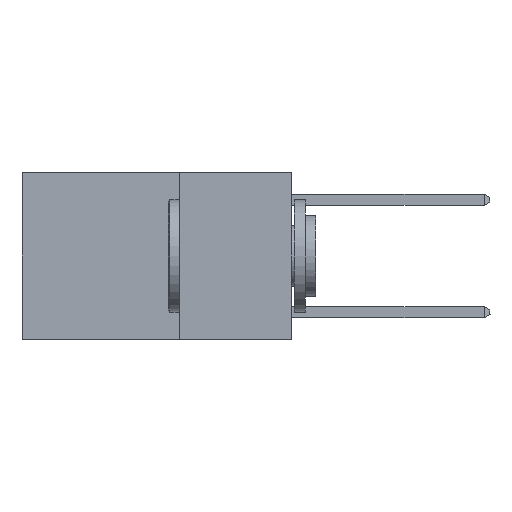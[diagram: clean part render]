
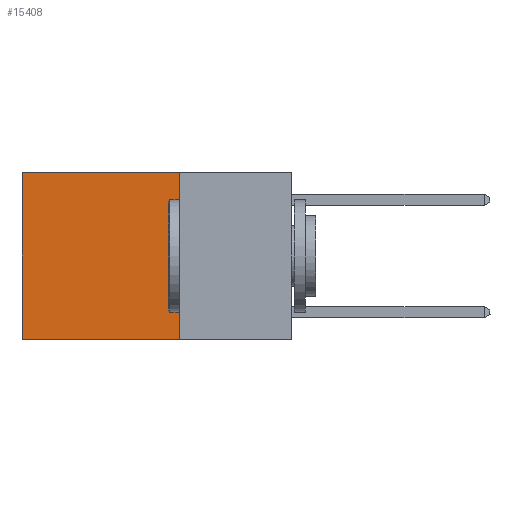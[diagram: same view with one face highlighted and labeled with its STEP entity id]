
A CAD part, left-side view. The second image highlights one B-rep face of the part: STEP entity #15408.
In plain terms, the highlighted planar face has unit normal (-1, 0, 0).
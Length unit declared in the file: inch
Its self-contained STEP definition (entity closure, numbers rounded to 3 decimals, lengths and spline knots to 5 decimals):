
#282 = VERTEX_POINT ( 'NONE', #19405 ) ;
#1904 = CARTESIAN_POINT ( 'NONE',  ( 0.2625, 0.25, -0.37 ) ) ;
#2249 = VECTOR ( 'NONE', #3381, 39.37008 ) ;
#2272 = LINE ( 'NONE', #5291, #2249 ) ;
#2725 = VERTEX_POINT ( 'NONE', #8084 ) ;
#3132 = VECTOR ( 'NONE', #20095, 39.37008 ) ;
#3381 = DIRECTION ( 'NONE',  ( 0., 0., -1. ) ) ;
#3656 = ORIENTED_EDGE ( 'NONE', *, *, #12179, .T. ) ;
#4263 = DIRECTION ( 'NONE',  ( 0., 0., -1. ) ) ;
#4786 = FACE_OUTER_BOUND ( 'NONE', #16411, .T. ) ;
#5291 = CARTESIAN_POINT ( 'NONE',  ( 0.2625, 0.6, 0. ) ) ;
#6138 = EDGE_CURVE ( 'NONE', #8339, #2725, #2272, .T. ) ;
#7059 = CARTESIAN_POINT ( 'NONE',  ( 0.2625, 0.25, 0. ) ) ;
#7097 = EDGE_CURVE ( 'NONE', #7276, #282, #9779, .T. ) ;
#7276 = VERTEX_POINT ( 'NONE', #9679 ) ;
#8084 = CARTESIAN_POINT ( 'NONE',  ( 0.2625, 0.6, -0.37 ) ) ;
#8153 = LINE ( 'NONE', #1904, #3132 ) ;
#8339 = VERTEX_POINT ( 'NONE', #14034 ) ;
#9037 = ORIENTED_EDGE ( 'NONE', *, *, #17999, .F. ) ;
#9679 = CARTESIAN_POINT ( 'NONE',  ( 0.2625, 0.25, 0. ) ) ;
#9779 = LINE ( 'NONE', #14354, #9848 ) ;
#9848 = VECTOR ( 'NONE', #4263, 39.37008 ) ;
#10473 = DIRECTION ( 'NONE',  ( 0., 0., -1. ) ) ;
#11497 = ORIENTED_EDGE ( 'NONE', *, *, #7097, .F. ) ;
#12179 = EDGE_CURVE ( 'NONE', #7276, #8339, #17061, .T. ) ;
#13060 = ORIENTED_EDGE ( 'NONE', *, *, #6138, .T. ) ;
#14034 = CARTESIAN_POINT ( 'NONE',  ( 0.2625, 0.6, 0. ) ) ;
#14354 = CARTESIAN_POINT ( 'NONE',  ( 0.2625, 0.25, 0. ) ) ;
#15408 = ADVANCED_FACE ( 'NONE', ( #4786 ), #17059, .F. ) ;
#16133 = CARTESIAN_POINT ( 'NONE',  ( 0.2625, 0.25, 0. ) ) ;
#16411 = EDGE_LOOP ( 'NONE', ( #13060, #9037, #11497, #3656 ) ) ;
#16556 = VECTOR ( 'NONE', #17784, 39.37008 ) ;
#17059 = PLANE ( 'NONE',  #20112 ) ;
#17061 = LINE ( 'NONE', #16133, #16556 ) ;
#17784 = DIRECTION ( 'NONE',  ( 0., 1., 0. ) ) ;
#17999 = EDGE_CURVE ( 'NONE', #282, #2725, #8153, .T. ) ;
#19405 = CARTESIAN_POINT ( 'NONE',  ( 0.2625, 0.25, -0.37 ) ) ;
#20095 = DIRECTION ( 'NONE',  ( 0., 1., 0. ) ) ;
#20112 = AXIS2_PLACEMENT_3D ( 'NONE', #7059, #20200, #10473 ) ;
#20200 = DIRECTION ( 'NONE',  ( 1., 0., 0. ) ) ;
